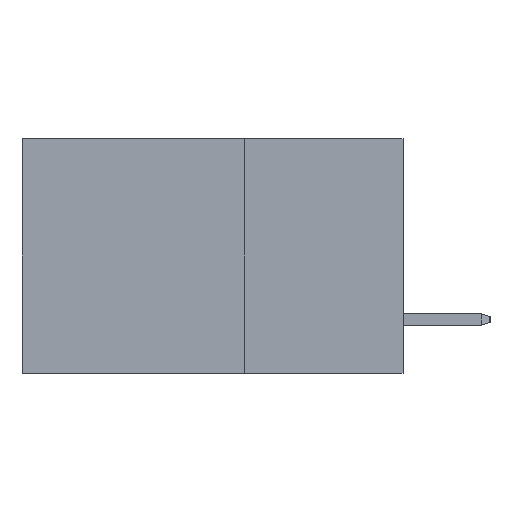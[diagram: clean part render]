
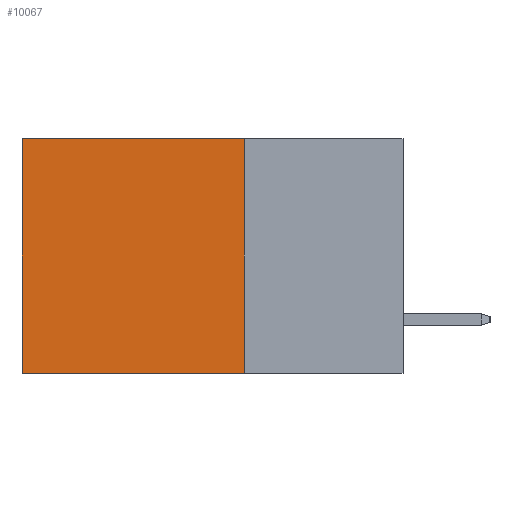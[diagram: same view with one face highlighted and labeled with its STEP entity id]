
A CAD part, left-side view. The second image highlights one B-rep face of the part: STEP entity #10067.
In plain terms, the highlighted planar face has unit normal (-1, 0, 0).
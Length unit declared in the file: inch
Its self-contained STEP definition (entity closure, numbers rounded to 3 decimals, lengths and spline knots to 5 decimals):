
#498 = DIRECTION ( 'NONE',  ( 0., 0., -1. ) ) ;
#1199 = VERTEX_POINT ( 'NONE', #11640 ) ;
#1319 = DIRECTION ( 'NONE',  ( 1., 0., 0. ) ) ;
#1483 = LINE ( 'NONE', #4439, #7461 ) ;
#1517 = ORIENTED_EDGE ( 'NONE', *, *, #5820, .F. ) ;
#1804 = LINE ( 'NONE', #5623, #7186 ) ;
#2258 = VERTEX_POINT ( 'NONE', #3819 ) ;
#3122 = ORIENTED_EDGE ( 'NONE', *, *, #4608, .F. ) ;
#3682 = VECTOR ( 'NONE', #8146, 39.37008 ) ;
#3792 = VERTEX_POINT ( 'NONE', #10846 ) ;
#3819 = CARTESIAN_POINT ( 'NONE',  ( 0.2875, 0.25, -0.37 ) ) ;
#4359 = VECTOR ( 'NONE', #498, 39.37008 ) ;
#4439 = CARTESIAN_POINT ( 'NONE',  ( 0.2875, 0.6, 0. ) ) ;
#4608 = EDGE_CURVE ( 'NONE', #3792, #2258, #5274, .T. ) ;
#5274 = LINE ( 'NONE', #8901, #4359 ) ;
#5382 = ORIENTED_EDGE ( 'NONE', *, *, #11036, .T. ) ;
#5623 = CARTESIAN_POINT ( 'NONE',  ( 0.2875, 0.25, -0.37 ) ) ;
#5820 = EDGE_CURVE ( 'NONE', #2258, #1199, #1804, .T. ) ;
#6334 = CARTESIAN_POINT ( 'NONE',  ( 0.2875, 0.6, 0. ) ) ;
#7033 = PLANE ( 'NONE',  #8286 ) ;
#7186 = VECTOR ( 'NONE', #7341, 39.37008 ) ;
#7328 = LINE ( 'NONE', #9049, #3682 ) ;
#7341 = DIRECTION ( 'NONE',  ( 0., 1., 0. ) ) ;
#7461 = VECTOR ( 'NONE', #10239, 39.37008 ) ;
#8146 = DIRECTION ( 'NONE',  ( 0., 1., 0. ) ) ;
#8286 = AXIS2_PLACEMENT_3D ( 'NONE', #10910, #1319, #9019 ) ;
#8325 = ORIENTED_EDGE ( 'NONE', *, *, #9243, .T. ) ;
#8710 = EDGE_LOOP ( 'NONE', ( #8325, #1517, #3122, #5382 ) ) ;
#8901 = CARTESIAN_POINT ( 'NONE',  ( 0.2875, 0.25, 0. ) ) ;
#9019 = DIRECTION ( 'NONE',  ( 0., 0., -1. ) ) ;
#9049 = CARTESIAN_POINT ( 'NONE',  ( 0.2875, 0.25, 0. ) ) ;
#9243 = EDGE_CURVE ( 'NONE', #10177, #1199, #1483, .T. ) ;
#10067 = ADVANCED_FACE ( 'NONE', ( #11856 ), #7033, .F. ) ;
#10177 = VERTEX_POINT ( 'NONE', #6334 ) ;
#10239 = DIRECTION ( 'NONE',  ( 0., 0., -1. ) ) ;
#10846 = CARTESIAN_POINT ( 'NONE',  ( 0.2875, 0.25, 0. ) ) ;
#10910 = CARTESIAN_POINT ( 'NONE',  ( 0.2875, 0.25, 0. ) ) ;
#11036 = EDGE_CURVE ( 'NONE', #3792, #10177, #7328, .T. ) ;
#11640 = CARTESIAN_POINT ( 'NONE',  ( 0.2875, 0.6, -0.37 ) ) ;
#11856 = FACE_OUTER_BOUND ( 'NONE', #8710, .T. ) ;
